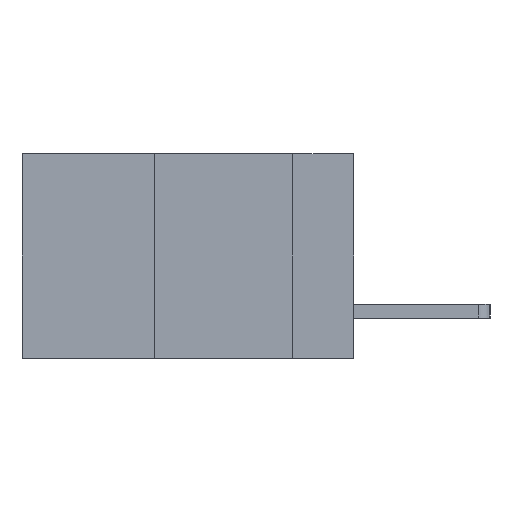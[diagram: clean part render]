
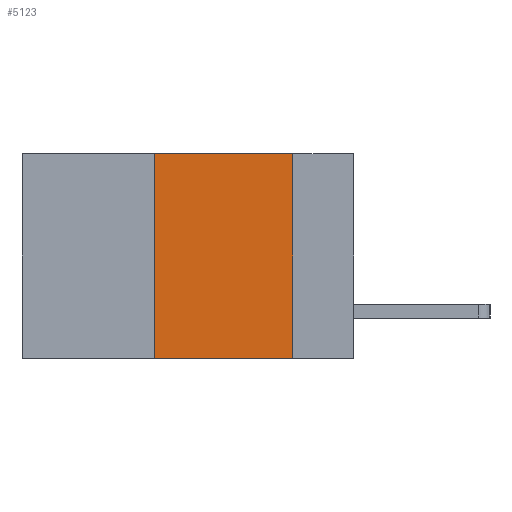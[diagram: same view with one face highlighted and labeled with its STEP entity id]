
A CAD part, left-side view. The second image highlights one B-rep face of the part: STEP entity #5123.
In plain terms, the highlighted planar face has unit normal (-1, 0, 0).
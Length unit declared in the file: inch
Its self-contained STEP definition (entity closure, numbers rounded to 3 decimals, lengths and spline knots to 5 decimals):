
#186 = LINE ( 'NONE', #11184, #6837 ) ;
#501 = VERTEX_POINT ( 'NONE', #971 ) ;
#971 = CARTESIAN_POINT ( 'NONE',  ( 0., 0.36, -0.37 ) ) ;
#1134 = CARTESIAN_POINT ( 'NONE',  ( 0., 0.36, 0. ) ) ;
#1314 = FACE_OUTER_BOUND ( 'NONE', #9399, .T. ) ;
#1439 = PLANE ( 'NONE',  #9968 ) ;
#1629 = LINE ( 'NONE', #2757, #2762 ) ;
#2116 = VERTEX_POINT ( 'NONE', #1134 ) ;
#2552 = CARTESIAN_POINT ( 'NONE',  ( 0., 0.11, -0.37 ) ) ;
#2757 = CARTESIAN_POINT ( 'NONE',  ( 0., 0.6, 0. ) ) ;
#2762 = VECTOR ( 'NONE', #3571, 39.37008 ) ;
#3383 = CARTESIAN_POINT ( 'NONE',  ( 0., 0.6, 0. ) ) ;
#3571 = DIRECTION ( 'NONE',  ( 0., -1., 0. ) ) ;
#3729 = CARTESIAN_POINT ( 'NONE',  ( 0., 0.6, -0.37 ) ) ;
#3803 = ORIENTED_EDGE ( 'NONE', *, *, #10322, .T. ) ;
#3944 = EDGE_CURVE ( 'NONE', #5169, #9362, #4445, .T. ) ;
#4445 = LINE ( 'NONE', #6492, #11627 ) ;
#5108 = DIRECTION ( 'NONE',  ( 0., 0., 1. ) ) ;
#5123 = ADVANCED_FACE ( 'NONE', ( #1314 ), #1439, .F. ) ;
#5169 = VERTEX_POINT ( 'NONE', #11395 ) ;
#5257 = EDGE_CURVE ( 'NONE', #2116, #5169, #1629, .T. ) ;
#5442 = DIRECTION ( 'NONE',  ( 1., 0., 0. ) ) ;
#6492 = CARTESIAN_POINT ( 'NONE',  ( 0., 0.11, 0. ) ) ;
#6837 = VECTOR ( 'NONE', #5108, 39.37008 ) ;
#7431 = DIRECTION ( 'NONE',  ( 0., 0., -1. ) ) ;
#8678 = ORIENTED_EDGE ( 'NONE', *, *, #5257, .F. ) ;
#9281 = EDGE_CURVE ( 'NONE', #501, #2116, #186, .T. ) ;
#9362 = VERTEX_POINT ( 'NONE', #2552 ) ;
#9399 = EDGE_LOOP ( 'NONE', ( #10191, #8678, #12084, #3803 ) ) ;
#9968 = AXIS2_PLACEMENT_3D ( 'NONE', #3383, #5442, #7431 ) ;
#10191 = ORIENTED_EDGE ( 'NONE', *, *, #3944, .F. ) ;
#10322 = EDGE_CURVE ( 'NONE', #501, #9362, #11608, .T. ) ;
#10734 = DIRECTION ( 'NONE',  ( 0., -1., 0. ) ) ;
#11184 = CARTESIAN_POINT ( 'NONE',  ( 0., 0.36, 0. ) ) ;
#11395 = CARTESIAN_POINT ( 'NONE',  ( 0., 0.11, 0. ) ) ;
#11522 = DIRECTION ( 'NONE',  ( 0., 0., -1. ) ) ;
#11608 = LINE ( 'NONE', #3729, #11931 ) ;
#11627 = VECTOR ( 'NONE', #11522, 39.37008 ) ;
#11931 = VECTOR ( 'NONE', #10734, 39.37008 ) ;
#12084 = ORIENTED_EDGE ( 'NONE', *, *, #9281, .F. ) ;
